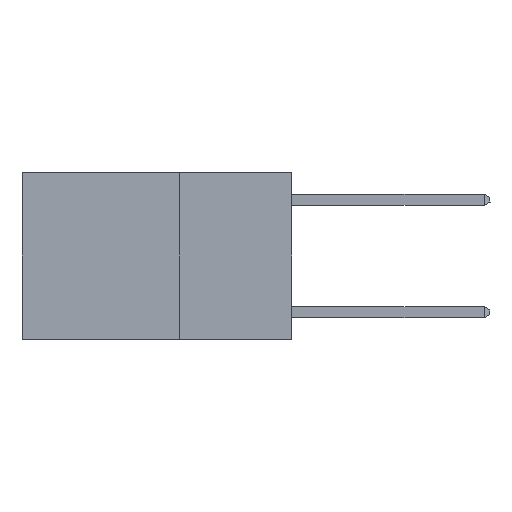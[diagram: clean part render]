
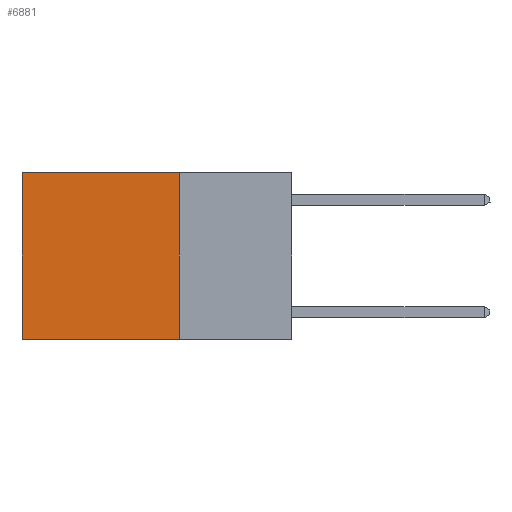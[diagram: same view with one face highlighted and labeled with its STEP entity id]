
A CAD part, left-side view. The second image highlights one B-rep face of the part: STEP entity #6881.
In plain terms, the highlighted planar face has unit normal (-1, 0, 0).
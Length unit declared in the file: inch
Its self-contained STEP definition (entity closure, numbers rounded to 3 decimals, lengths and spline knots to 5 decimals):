
#236 = EDGE_CURVE ( 'NONE', #16101, #9563, #13937, .T. ) ;
#1149 = VECTOR ( 'NONE', #4847, 39.37008 ) ;
#1159 = DIRECTION ( 'NONE',  ( 0., 0., -1. ) ) ;
#1850 = VECTOR ( 'NONE', #9940, 39.37008 ) ;
#2964 = ORIENTED_EDGE ( 'NONE', *, *, #236, .F. ) ;
#3611 = FACE_OUTER_BOUND ( 'NONE', #15780, .T. ) ;
#3815 = LINE ( 'NONE', #6779, #1850 ) ;
#4559 = VERTEX_POINT ( 'NONE', #4966 ) ;
#4847 = DIRECTION ( 'NONE',  ( 0., 1., 0. ) ) ;
#4966 = CARTESIAN_POINT ( 'NONE',  ( 0.2625, 0.6, 0. ) ) ;
#5920 = EDGE_CURVE ( 'NONE', #7020, #16101, #3815, .T. ) ;
#6779 = CARTESIAN_POINT ( 'NONE',  ( 0.2625, 0.25, 0. ) ) ;
#6873 = ORIENTED_EDGE ( 'NONE', *, *, #17643, .T. ) ;
#6881 = ADVANCED_FACE ( 'NONE', ( #3611 ), #15538, .F. ) ;
#7020 = VERTEX_POINT ( 'NONE', #9926 ) ;
#8456 = VECTOR ( 'NONE', #12786, 39.37008 ) ;
#9458 = LINE ( 'NONE', #17585, #11461 ) ;
#9563 = VERTEX_POINT ( 'NONE', #12243 ) ;
#9604 = DIRECTION ( 'NONE',  ( 1., 0., 0. ) ) ;
#9926 = CARTESIAN_POINT ( 'NONE',  ( 0.2625, 0.25, 0. ) ) ;
#9940 = DIRECTION ( 'NONE',  ( 0., 0., -1. ) ) ;
#10086 = CARTESIAN_POINT ( 'NONE',  ( 0.2625, 0.6, 0. ) ) ;
#10433 = ORIENTED_EDGE ( 'NONE', *, *, #15165, .T. ) ;
#10919 = AXIS2_PLACEMENT_3D ( 'NONE', #18034, #9604, #1159 ) ;
#11461 = VECTOR ( 'NONE', #14960, 39.37008 ) ;
#11734 = CARTESIAN_POINT ( 'NONE',  ( 0.2625, 0.25, -0.37 ) ) ;
#12223 = LINE ( 'NONE', #10086, #8456 ) ;
#12243 = CARTESIAN_POINT ( 'NONE',  ( 0.2625, 0.6, -0.37 ) ) ;
#12786 = DIRECTION ( 'NONE',  ( 0., 0., -1. ) ) ;
#13937 = LINE ( 'NONE', #17473, #1149 ) ;
#13990 = ORIENTED_EDGE ( 'NONE', *, *, #5920, .F. ) ;
#14960 = DIRECTION ( 'NONE',  ( 0., 1., 0. ) ) ;
#15165 = EDGE_CURVE ( 'NONE', #4559, #9563, #12223, .T. ) ;
#15538 = PLANE ( 'NONE',  #10919 ) ;
#15780 = EDGE_LOOP ( 'NONE', ( #10433, #2964, #13990, #6873 ) ) ;
#16101 = VERTEX_POINT ( 'NONE', #11734 ) ;
#17473 = CARTESIAN_POINT ( 'NONE',  ( 0.2625, 0.25, -0.37 ) ) ;
#17585 = CARTESIAN_POINT ( 'NONE',  ( 0.2625, 0.25, 0. ) ) ;
#17643 = EDGE_CURVE ( 'NONE', #7020, #4559, #9458, .T. ) ;
#18034 = CARTESIAN_POINT ( 'NONE',  ( 0.2625, 0.25, 0. ) ) ;
